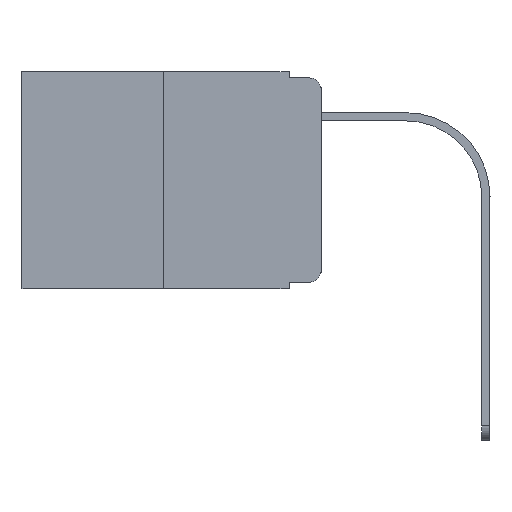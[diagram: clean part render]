
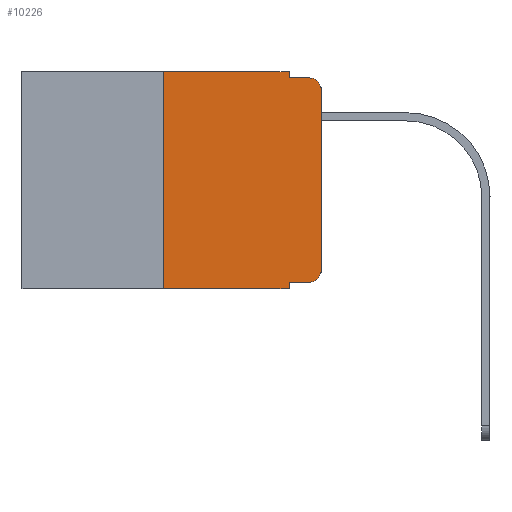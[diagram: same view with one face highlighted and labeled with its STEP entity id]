
A CAD part, left-side view. The second image highlights one B-rep face of the part: STEP entity #10226.
In plain terms, the highlighted planar face has unit normal (-1, 0, 0).
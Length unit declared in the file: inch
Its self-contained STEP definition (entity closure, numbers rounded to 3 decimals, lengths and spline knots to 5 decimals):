
#107 = CARTESIAN_POINT ( 'NONE',  ( 0., 0., -0.313 ) ) ;
#274 = CARTESIAN_POINT ( 'NONE',  ( 0., 0.473, -0.343 ) ) ;
#342 = ORIENTED_EDGE ( 'NONE', *, *, #11677, .F. ) ;
#1544 = ORIENTED_EDGE ( 'NONE', *, *, #10423, .T. ) ;
#1573 = CARTESIAN_POINT ( 'NONE',  ( 0., 0., -0.03 ) ) ;
#2054 = CARTESIAN_POINT ( 'NONE',  ( 0., 0.473, 0. ) ) ;
#2066 = ORIENTED_EDGE ( 'NONE', *, *, #6701, .T. ) ;
#2464 = DIRECTION ( 'NONE',  ( 0., 0., -1. ) ) ;
#2472 = CARTESIAN_POINT ( 'NONE',  ( 0., 0.25, 0. ) ) ;
#2834 = DIRECTION ( 'NONE',  ( -1., 0., 0. ) ) ;
#2855 = VERTEX_POINT ( 'NONE', #12853 ) ;
#2877 = VERTEX_POINT ( 'NONE', #9162 ) ;
#3051 = EDGE_LOOP ( 'NONE', ( #3523, #2066, #342, #6577, #17315, #11039, #1544, #4416, #6293, #14178 ) ) ;
#3075 = VECTOR ( 'NONE', #13527, 39.37008 ) ;
#3296 = AXIS2_PLACEMENT_3D ( 'NONE', #2054, #17434, #4826 ) ;
#3392 = DIRECTION ( 'NONE',  ( 0., 0., 1. ) ) ;
#3430 = PLANE ( 'NONE',  #3296 ) ;
#3459 = VECTOR ( 'NONE', #16319, 39.37008 ) ;
#3523 = ORIENTED_EDGE ( 'NONE', *, *, #6468, .T. ) ;
#3573 = CARTESIAN_POINT ( 'NONE',  ( 0., 0., 0. ) ) ;
#3661 = VECTOR ( 'NONE', #3392, 39.37008 ) ;
#3910 = DIRECTION ( 'NONE',  ( 0., -1., 0. ) ) ;
#4014 = LINE ( 'NONE', #15337, #8925 ) ;
#4416 = ORIENTED_EDGE ( 'NONE', *, *, #17681, .F. ) ;
#4826 = DIRECTION ( 'NONE',  ( 0., 0., -1. ) ) ;
#5232 = VECTOR ( 'NONE', #3910, 39.37008 ) ;
#5249 = LINE ( 'NONE', #10854, #11603 ) ;
#5382 = DIRECTION ( 'NONE',  ( -1., 0., 0. ) ) ;
#5421 = CIRCLE ( 'NONE', #12180, 0.02 ) ;
#5460 = LINE ( 'NONE', #16583, #3459 ) ;
#5571 = DIRECTION ( 'NONE',  ( 0., 0., -1. ) ) ;
#5838 = VERTEX_POINT ( 'NONE', #7116 ) ;
#6293 = ORIENTED_EDGE ( 'NONE', *, *, #11137, .T. ) ;
#6468 = EDGE_CURVE ( 'NONE', #8847, #13036, #16004, .T. ) ;
#6518 = EDGE_CURVE ( 'NONE', #16449, #12034, #9485, .T. ) ;
#6577 = ORIENTED_EDGE ( 'NONE', *, *, #12498, .F. ) ;
#6701 = EDGE_CURVE ( 'NONE', #13036, #11483, #18122, .T. ) ;
#7116 = CARTESIAN_POINT ( 'NONE',  ( 0., 0.051, 0. ) ) ;
#8065 = CARTESIAN_POINT ( 'NONE',  ( 0., 0.473, 0. ) ) ;
#8213 = CARTESIAN_POINT ( 'NONE',  ( 0., 0.25, 0. ) ) ;
#8847 = VERTEX_POINT ( 'NONE', #107 ) ;
#8925 = VECTOR ( 'NONE', #11012, 39.37008 ) ;
#9108 = LINE ( 'NONE', #274, #13039 ) ;
#9162 = CARTESIAN_POINT ( 'NONE',  ( 0., 0.051, -0.333 ) ) ;
#9485 = LINE ( 'NONE', #2472, #3075 ) ;
#9961 = DIRECTION ( 'NONE',  ( 0., -1., 0. ) ) ;
#10189 = AXIS2_PLACEMENT_3D ( 'NONE', #11574, #2834, #14241 ) ;
#10226 = ADVANCED_FACE ( 'NONE', ( #11819 ), #3430, .F. ) ;
#10423 = EDGE_CURVE ( 'NONE', #16449, #2855, #9108, .T. ) ;
#10838 = CARTESIAN_POINT ( 'NONE',  ( 0., 0.02, -0.333 ) ) ;
#10854 = CARTESIAN_POINT ( 'NONE',  ( 0., 0.051, 0. ) ) ;
#11012 = DIRECTION ( 'NONE',  ( 0., -1., 0. ) ) ;
#11039 = ORIENTED_EDGE ( 'NONE', *, *, #6518, .F. ) ;
#11137 = EDGE_CURVE ( 'NONE', #2877, #14232, #4014, .T. ) ;
#11483 = VERTEX_POINT ( 'NONE', #12099 ) ;
#11547 = EDGE_CURVE ( 'NONE', #14232, #8847, #5421, .T. ) ;
#11574 = CARTESIAN_POINT ( 'NONE',  ( 0., 0.02, -0.03 ) ) ;
#11603 = VECTOR ( 'NONE', #2464, 39.37008 ) ;
#11677 = EDGE_CURVE ( 'NONE', #12177, #11483, #12373, .T. ) ;
#11819 = FACE_OUTER_BOUND ( 'NONE', #3051, .T. ) ;
#12034 = VERTEX_POINT ( 'NONE', #8213 ) ;
#12099 = CARTESIAN_POINT ( 'NONE',  ( 0., 0.02, -0.01 ) ) ;
#12177 = VERTEX_POINT ( 'NONE', #13071 ) ;
#12180 = AXIS2_PLACEMENT_3D ( 'NONE', #17623, #5382, #5571 ) ;
#12373 = LINE ( 'NONE', #12550, #15977 ) ;
#12461 = DIRECTION ( 'NONE',  ( 0., -1., 0. ) ) ;
#12498 = EDGE_CURVE ( 'NONE', #5838, #12177, #5249, .T. ) ;
#12550 = CARTESIAN_POINT ( 'NONE',  ( 0., 0.051, -0.01 ) ) ;
#12853 = CARTESIAN_POINT ( 'NONE',  ( 0., 0.051, -0.343 ) ) ;
#13036 = VERTEX_POINT ( 'NONE', #1573 ) ;
#13039 = VECTOR ( 'NONE', #9961, 39.37008 ) ;
#13071 = CARTESIAN_POINT ( 'NONE',  ( 0., 0.051, -0.01 ) ) ;
#13527 = DIRECTION ( 'NONE',  ( 0., 0., 1. ) ) ;
#14002 = CARTESIAN_POINT ( 'NONE',  ( 0., 0.25, -0.343 ) ) ;
#14178 = ORIENTED_EDGE ( 'NONE', *, *, #11547, .T. ) ;
#14232 = VERTEX_POINT ( 'NONE', #10838 ) ;
#14241 = DIRECTION ( 'NONE',  ( 0., 0., -1. ) ) ;
#15337 = CARTESIAN_POINT ( 'NONE',  ( 0., 0.051, -0.333 ) ) ;
#15819 = EDGE_CURVE ( 'NONE', #12034, #5838, #16056, .T. ) ;
#15977 = VECTOR ( 'NONE', #12461, 39.37008 ) ;
#16004 = LINE ( 'NONE', #3573, #3661 ) ;
#16056 = LINE ( 'NONE', #8065, #5232 ) ;
#16319 = DIRECTION ( 'NONE',  ( 0., 0., -1. ) ) ;
#16449 = VERTEX_POINT ( 'NONE', #14002 ) ;
#16583 = CARTESIAN_POINT ( 'NONE',  ( 0., 0.051, 0. ) ) ;
#17315 = ORIENTED_EDGE ( 'NONE', *, *, #15819, .F. ) ;
#17434 = DIRECTION ( 'NONE',  ( 1., 0., 0. ) ) ;
#17623 = CARTESIAN_POINT ( 'NONE',  ( 0., 0.02, -0.313 ) ) ;
#17681 = EDGE_CURVE ( 'NONE', #2877, #2855, #5460, .T. ) ;
#18122 = CIRCLE ( 'NONE', #10189, 0.02 ) ;
